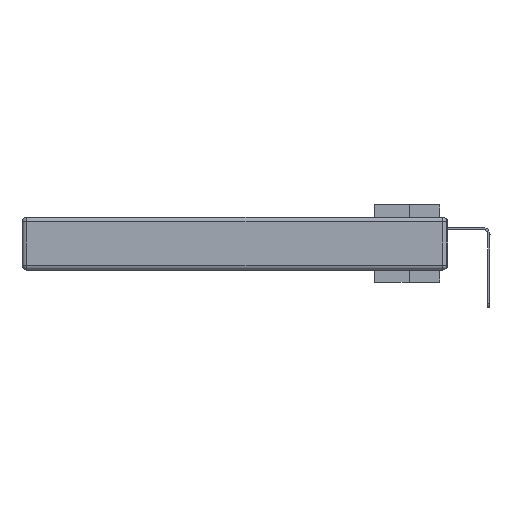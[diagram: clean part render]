
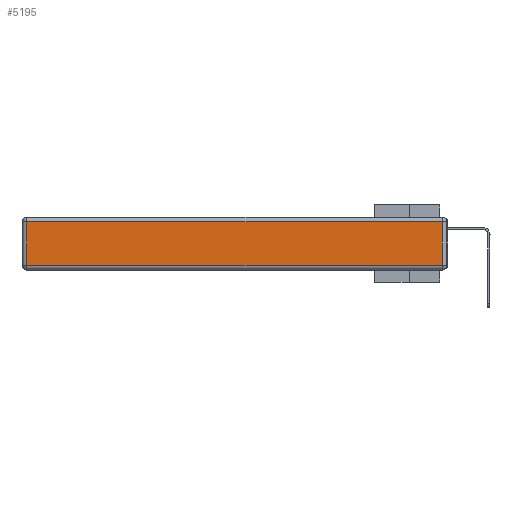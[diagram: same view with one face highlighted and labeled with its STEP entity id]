
A CAD part, left-side view. The second image highlights one B-rep face of the part: STEP entity #5195.
In plain terms, the highlighted planar face has unit normal (-1, 0, 0).
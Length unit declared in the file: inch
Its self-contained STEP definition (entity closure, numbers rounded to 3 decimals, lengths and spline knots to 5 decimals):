
#771 = CARTESIAN_POINT ( 'NONE',  ( 0., 2.75, -0.03 ) ) ;
#1404 = PLANE ( 'NONE',  #12627 ) ;
#4491 = DIRECTION ( 'NONE',  ( 0., -1., 0. ) ) ;
#5195 = ADVANCED_FACE ( 'NONE', ( #30622 ), #1404, .T. ) ;
#5603 = EDGE_CURVE ( 'NONE', #10871, #34919, #18839, .T. ) ;
#6616 = VERTEX_POINT ( 'NONE', #20442 ) ;
#7171 = ORIENTED_EDGE ( 'NONE', *, *, #12044, .T. ) ;
#7654 = CARTESIAN_POINT ( 'NONE',  ( 0., 0., -0.343 ) ) ;
#9600 = VECTOR ( 'NONE', #31628, 39.37008 ) ;
#9882 = DIRECTION ( 'NONE',  ( 0., 1., 0. ) ) ;
#10767 = LINE ( 'NONE', #23369, #30336 ) ;
#10871 = VERTEX_POINT ( 'NONE', #32322 ) ;
#11060 = CARTESIAN_POINT ( 'NONE',  ( 0., 0.03, -0.03 ) ) ;
#12044 = EDGE_CURVE ( 'NONE', #24640, #10871, #13089, .T. ) ;
#12627 = AXIS2_PLACEMENT_3D ( 'NONE', #7654, #13912, #38835 ) ;
#13089 = LINE ( 'NONE', #771, #30228 ) ;
#13912 = DIRECTION ( 'NONE',  ( -1., 0., 0. ) ) ;
#14100 = DIRECTION ( 'NONE',  ( 0., 0., 1. ) ) ;
#18839 = LINE ( 'NONE', #35822, #9600 ) ;
#20442 = CARTESIAN_POINT ( 'NONE',  ( 0., 0.03, -0.313 ) ) ;
#23369 = CARTESIAN_POINT ( 'NONE',  ( 0., 0.03, -0.343 ) ) ;
#24640 = VERTEX_POINT ( 'NONE', #11060 ) ;
#25020 = ORIENTED_EDGE ( 'NONE', *, *, #37834, .T. ) ;
#25832 = CARTESIAN_POINT ( 'NONE',  ( 0., 0., -0.313 ) ) ;
#26138 = ORIENTED_EDGE ( 'NONE', *, *, #28905, .T. ) ;
#26467 = ORIENTED_EDGE ( 'NONE', *, *, #5603, .T. ) ;
#28905 = EDGE_CURVE ( 'NONE', #6616, #24640, #10767, .T. ) ;
#30228 = VECTOR ( 'NONE', #9882, 39.37008 ) ;
#30336 = VECTOR ( 'NONE', #14100, 39.37008 ) ;
#30622 = FACE_OUTER_BOUND ( 'NONE', #33979, .T. ) ;
#30817 = VECTOR ( 'NONE', #4491, 39.37008 ) ;
#31628 = DIRECTION ( 'NONE',  ( 0., 0., -1. ) ) ;
#32322 = CARTESIAN_POINT ( 'NONE',  ( 0., 2.72, -0.03 ) ) ;
#33979 = EDGE_LOOP ( 'NONE', ( #25020, #26138, #7171, #26467 ) ) ;
#34919 = VERTEX_POINT ( 'NONE', #35764 ) ;
#35764 = CARTESIAN_POINT ( 'NONE',  ( 0., 2.72, -0.313 ) ) ;
#35822 = CARTESIAN_POINT ( 'NONE',  ( 0., 2.72, -0.343 ) ) ;
#37103 = LINE ( 'NONE', #25832, #30817 ) ;
#37834 = EDGE_CURVE ( 'NONE', #34919, #6616, #37103, .T. ) ;
#38835 = DIRECTION ( 'NONE',  ( 0., 0., 1. ) ) ;
